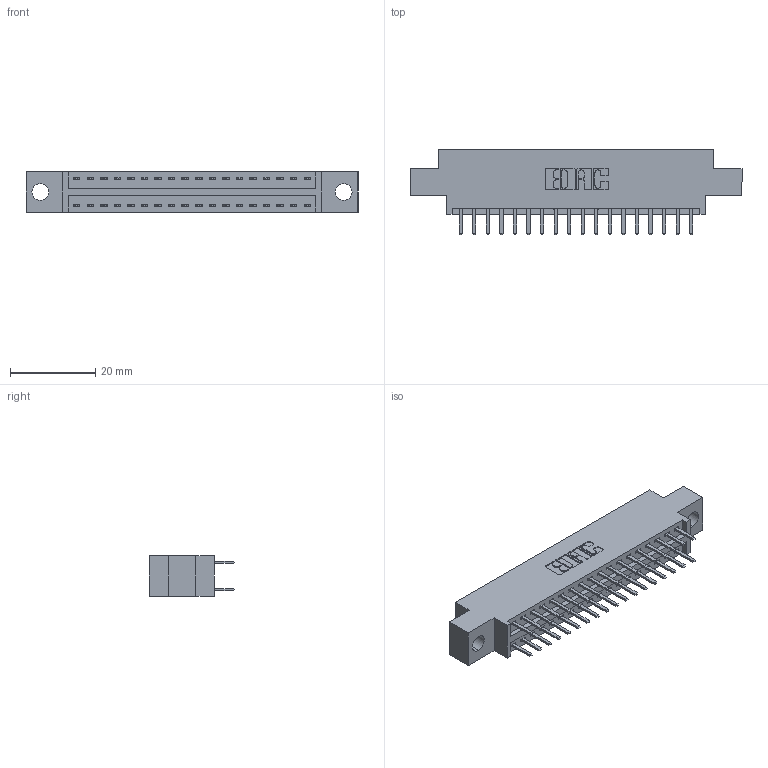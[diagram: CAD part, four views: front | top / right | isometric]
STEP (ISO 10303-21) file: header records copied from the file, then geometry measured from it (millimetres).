
FILE_DESCRIPTION (( 'STEP AP203' ), '1' );
FILE_NAME ('346-036-520-804.STEP', '2022-05-19T21:01:18', ( '' ), ( '' ), 'SwSTEP 2.0', 'SolidWorks 2020', '' );
FILE_SCHEMA (( 'CONFIG_CONTROL_DESIGN' ));
Length unit declared in the file: inch
Products named in the file (3): 346-036-520-804; 346 Part_0.170 Offset - 0.156 Dia-TH; 345-292-001_345-293-120
Assembly tree (37 placements, depth 2):
  346-036-520-804
    346 Part_0.170 Offset - 0.156 Dia-TH
    345-292-001_345-293-120  x36
Bounding box: 77.72 x 20.02 x 9.4 mm (x, y, z)
Volume: 7116.3 mm3; surface area: 9395 mm2
Topology: 37 solids, 37 shells, 2156 faces, 6245 edges, 4066 vertices
Faces by surface type: plane 1426, cylinder 730
Entity records: 15643 total; most frequent: CARTESIAN_POINT 2630, ORIENTED_EDGE 2550, DIRECTION 2355, EDGE_CURVE 1275, VECTOR 1067, LINE 1067, VERTEX_POINT 846, AXIS2_PLACEMENT_3D 644
